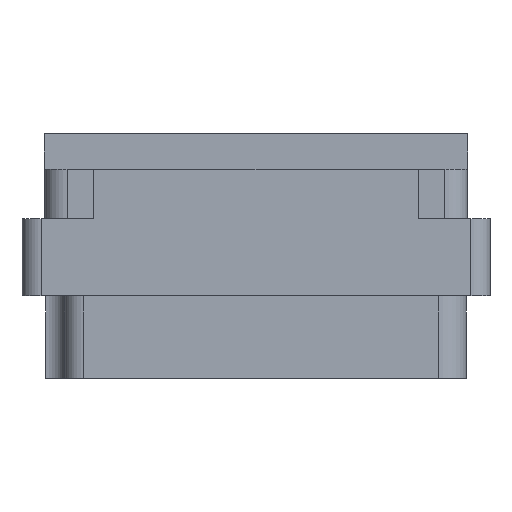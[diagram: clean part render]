
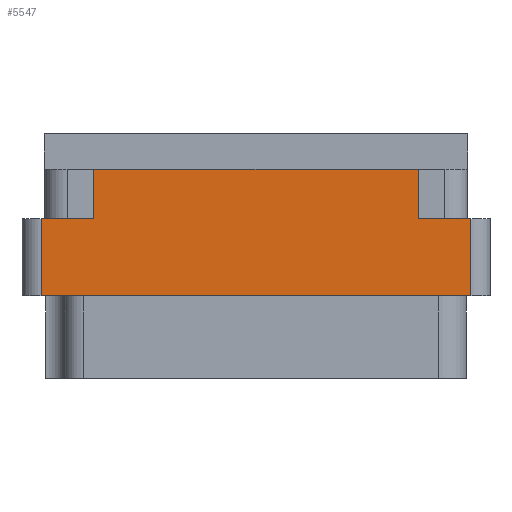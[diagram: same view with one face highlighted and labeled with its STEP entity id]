
A CAD part, left-side view. The second image highlights one B-rep face of the part: STEP entity #5547.
In plain terms, the highlighted planar face has unit normal (-1, 0, 0).
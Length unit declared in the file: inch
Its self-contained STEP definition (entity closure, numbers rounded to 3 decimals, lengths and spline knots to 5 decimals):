
#654 = LINE ( 'NONE', #5058, #66697 ) ;
#1753 = EDGE_CURVE ( 'NONE', #6400, #73197, #4791, .T. ) ;
#2772 = VECTOR ( 'NONE', #23141, 39.37008 ) ;
#3485 = VECTOR ( 'NONE', #42731, 39.37008 ) ;
#4791 = LINE ( 'NONE', #65911, #2772 ) ;
#5058 = CARTESIAN_POINT ( 'NONE',  ( -1.375, -0.7005, -0.798 ) ) ;
#5347 = DIRECTION ( 'NONE',  ( 0., 0., 1. ) ) ;
#5547 = ADVANCED_FACE ( 'NONE', ( #78007 ), #26390, .T. ) ;
#6060 = VERTEX_POINT ( 'NONE', #48452 ) ;
#6400 = VERTEX_POINT ( 'NONE', #80206 ) ;
#6745 = ORIENTED_EDGE ( 'NONE', *, *, #51552, .T. ) ;
#7918 = EDGE_CURVE ( 'NONE', #75758, #6060, #17731, .T. ) ;
#9139 = EDGE_LOOP ( 'NONE', ( #25874, #6745, #82957, #15735, #11265, #37550, #40889, #20509 ) ) ;
#10200 = VECTOR ( 'NONE', #22855, 39.37008 ) ;
#11265 = ORIENTED_EDGE ( 'NONE', *, *, #46138, .F. ) ;
#11590 = VECTOR ( 'NONE', #44758, 39.37008 ) ;
#15037 = DIRECTION ( 'NONE',  ( -1., 0., 0. ) ) ;
#15735 = ORIENTED_EDGE ( 'NONE', *, *, #29861, .T. ) ;
#17731 = LINE ( 'NONE', #35643, #3485 ) ;
#18551 = LINE ( 'NONE', #30512, #33806 ) ;
#18677 = AXIS2_PLACEMENT_3D ( 'NONE', #47686, #15037, #66701 ) ;
#20509 = ORIENTED_EDGE ( 'NONE', *, *, #43788, .F. ) ;
#21981 = DIRECTION ( 'NONE',  ( 0., 0., 1. ) ) ;
#22855 = DIRECTION ( 'NONE',  ( 0., 1., 0. ) ) ;
#23141 = DIRECTION ( 'NONE',  ( 0., -1., 0. ) ) ;
#25874 = ORIENTED_EDGE ( 'NONE', *, *, #1753, .F. ) ;
#26390 = PLANE ( 'NONE',  #18677 ) ;
#28543 = CARTESIAN_POINT ( 'NONE',  ( -1.375, -0.7005, -0.529 ) ) ;
#29861 = EDGE_CURVE ( 'NONE', #34808, #58713, #654, .T. ) ;
#30512 = CARTESIAN_POINT ( 'NONE',  ( -1.375, 0., -0.277 ) ) ;
#33806 = VECTOR ( 'NONE', #69456, 39.37008 ) ;
#34808 = VERTEX_POINT ( 'NONE', #28543 ) ;
#35643 = CARTESIAN_POINT ( 'NONE',  ( -1.375, 0.7625, -0.117 ) ) ;
#37550 = ORIENTED_EDGE ( 'NONE', *, *, #45353, .T. ) ;
#39107 = EDGE_CURVE ( 'NONE', #34808, #65409, #46790, .T. ) ;
#40889 = ORIENTED_EDGE ( 'NONE', *, *, #7918, .F. ) ;
#42731 = DIRECTION ( 'NONE',  ( 0., -1., 0. ) ) ;
#43788 = EDGE_CURVE ( 'NONE', #73197, #75758, #80014, .T. ) ;
#44475 = CARTESIAN_POINT ( 'NONE',  ( -1.375, 0.7005, -0.798 ) ) ;
#44758 = DIRECTION ( 'NONE',  ( 0., 0., -1. ) ) ;
#45353 = EDGE_CURVE ( 'NONE', #75717, #6060, #49000, .T. ) ;
#45460 = CARTESIAN_POINT ( 'NONE',  ( -1.375, 0.5285, -0.277 ) ) ;
#46138 = EDGE_CURVE ( 'NONE', #75717, #58713, #18551, .T. ) ;
#46790 = LINE ( 'NONE', #47927, #10200 ) ;
#47686 = CARTESIAN_POINT ( 'NONE',  ( -1.375, -0.7625, -0.798 ) ) ;
#47927 = CARTESIAN_POINT ( 'NONE',  ( -1.375, 0., -0.529 ) ) ;
#48452 = CARTESIAN_POINT ( 'NONE',  ( -1.375, -0.5285, -0.117 ) ) ;
#49000 = LINE ( 'NONE', #53945, #55010 ) ;
#50207 = LINE ( 'NONE', #44475, #11590 ) ;
#50928 = CARTESIAN_POINT ( 'NONE',  ( -1.375, -0.5285, -0.277 ) ) ;
#51552 = EDGE_CURVE ( 'NONE', #6400, #65409, #50207, .T. ) ;
#53945 = CARTESIAN_POINT ( 'NONE',  ( -1.375, -0.5285, -0.277 ) ) ;
#54581 = CARTESIAN_POINT ( 'NONE',  ( -1.375, -0.7005, -0.277 ) ) ;
#55010 = VECTOR ( 'NONE', #73475, 39.37008 ) ;
#55919 = CARTESIAN_POINT ( 'NONE',  ( -1.375, 0.5285, -0.277 ) ) ;
#58713 = VERTEX_POINT ( 'NONE', #54581 ) ;
#65409 = VERTEX_POINT ( 'NONE', #79213 ) ;
#65911 = CARTESIAN_POINT ( 'NONE',  ( -1.375, 0., -0.277 ) ) ;
#66697 = VECTOR ( 'NONE', #5347, 39.37008 ) ;
#66701 = DIRECTION ( 'NONE',  ( 0., 0., 1. ) ) ;
#69456 = DIRECTION ( 'NONE',  ( 0., -1., 0. ) ) ;
#73197 = VERTEX_POINT ( 'NONE', #55919 ) ;
#73475 = DIRECTION ( 'NONE',  ( 0., 0., 1. ) ) ;
#75717 = VERTEX_POINT ( 'NONE', #50928 ) ;
#75758 = VERTEX_POINT ( 'NONE', #76920 ) ;
#76920 = CARTESIAN_POINT ( 'NONE',  ( -1.375, 0.5285, -0.117 ) ) ;
#77983 = VECTOR ( 'NONE', #21981, 39.37008 ) ;
#78007 = FACE_OUTER_BOUND ( 'NONE', #9139, .T. ) ;
#79213 = CARTESIAN_POINT ( 'NONE',  ( -1.375, 0.7005, -0.529 ) ) ;
#80014 = LINE ( 'NONE', #45460, #77983 ) ;
#80206 = CARTESIAN_POINT ( 'NONE',  ( -1.375, 0.7005, -0.277 ) ) ;
#82957 = ORIENTED_EDGE ( 'NONE', *, *, #39107, .F. ) ;
